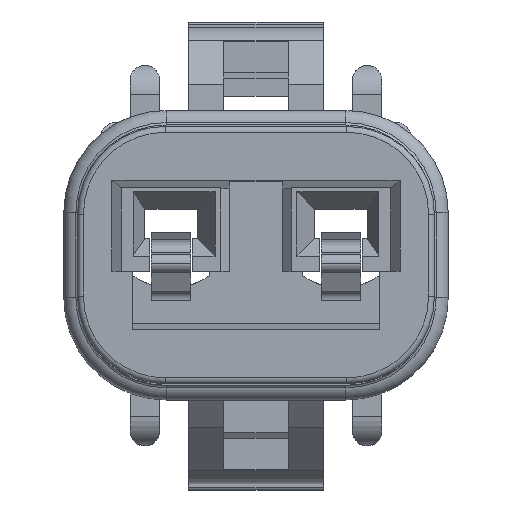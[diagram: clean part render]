
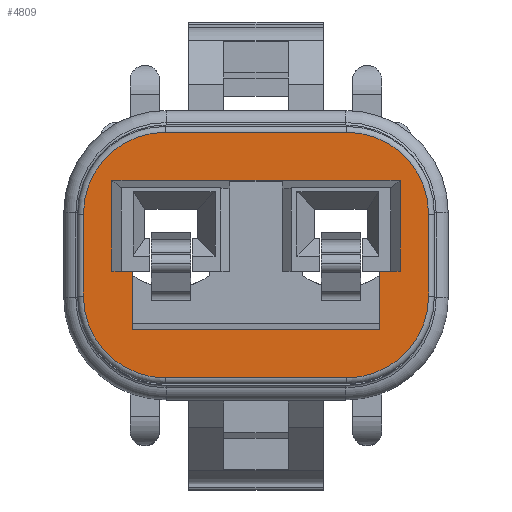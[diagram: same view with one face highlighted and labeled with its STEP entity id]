
A CAD part, top view. The second image highlights one B-rep face of the part: STEP entity #4809.
In plain terms, the highlighted planar face has unit normal (0, 0, 1).
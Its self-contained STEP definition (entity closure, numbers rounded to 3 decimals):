
#49 = ORIENTED_EDGE ( 'NONE', *, *, #10752, .T. ) ;
#76 = ORIENTED_EDGE ( 'NONE', *, *, #14027, .T. ) ;
#453 = CARTESIAN_POINT ( 'NONE',  ( -4.925, 2.55, 1.2 ) ) ;
#725 = DIRECTION ( 'NONE',  ( 0., -1., 0. ) ) ;
#781 = VERTEX_POINT ( 'NONE', #19091 ) ;
#872 = FACE_OUTER_BOUND ( 'NONE', #15510, .T. ) ;
#918 = CIRCLE ( 'NONE', #20754, 2.8 ) ;
#1000 = LINE ( 'NONE', #7420, #5694 ) ;
#1250 = DIRECTION ( 'NONE',  ( 0., 1., 0. ) ) ;
#1324 = VERTEX_POINT ( 'NONE', #19499 ) ;
#1380 = DIRECTION ( 'NONE',  ( -1., 0., 0. ) ) ;
#1539 = DIRECTION ( 'NONE',  ( 0., 1., 0. ) ) ;
#1746 = VERTEX_POINT ( 'NONE', #6311 ) ;
#1815 = VERTEX_POINT ( 'NONE', #8735 ) ;
#2242 = ORIENTED_EDGE ( 'NONE', *, *, #15572, .T. ) ;
#2269 = EDGE_CURVE ( 'NONE', #15715, #1746, #9987, .T. ) ;
#2289 = DIRECTION ( 'NONE',  ( -1., 0., 0. ) ) ;
#2416 = EDGE_CURVE ( 'NONE', #15825, #19016, #18409, .T. ) ;
#2464 = DIRECTION ( 'NONE',  ( 0., -1., 0. ) ) ;
#2472 = DIRECTION ( 'NONE',  ( 0., 0., 1. ) ) ;
#2514 = CARTESIAN_POINT ( 'NONE',  ( -3.1, -1.4, 1.2 ) ) ;
#2639 = CARTESIAN_POINT ( 'NONE',  ( 3.1, 4.2, 1.2 ) ) ;
#2837 = AXIS2_PLACEMENT_3D ( 'NONE', #20809, #11456, #12719 ) ;
#3070 = LINE ( 'NONE', #6118, #18614 ) ;
#3193 = CARTESIAN_POINT ( 'NONE',  ( 3.1, 4.2, 1.2 ) ) ;
#3314 = CARTESIAN_POINT ( 'NONE',  ( 3.1, -4.2, 1.2 ) ) ;
#3358 = CARTESIAN_POINT ( 'NONE',  ( -0.9, 2.55, 1.2 ) ) ;
#3387 = LINE ( 'NONE', #9812, #15746 ) ;
#3481 = EDGE_LOOP ( 'NONE', ( #18229, #16703, #19898, #76, #18916, #15585, #14771, #2242, #17295, #3567 ) ) ;
#3567 = ORIENTED_EDGE ( 'NONE', *, *, #6371, .T. ) ;
#3836 = DIRECTION ( 'NONE',  ( 1., 0., 0. ) ) ;
#4118 = EDGE_CURVE ( 'NONE', #15641, #1815, #9157, .T. ) ;
#4176 = VERTEX_POINT ( 'NONE', #8186 ) ;
#4182 = CARTESIAN_POINT ( 'NONE',  ( -4.225, -0.55, 1.2 ) ) ;
#4259 = AXIS2_PLACEMENT_3D ( 'NONE', #2514, #10612, #16950 ) ;
#4262 = CARTESIAN_POINT ( 'NONE',  ( 0., 0., 1.2 ) ) ;
#4807 = CARTESIAN_POINT ( 'NONE',  ( -4.225, -2.55, 1.2 ) ) ;
#4809 = ADVANCED_FACE ( 'NONE', ( #15211, #872 ), #9203, .T. ) ;
#4913 = VERTEX_POINT ( 'NONE', #3193 ) ;
#5470 = VECTOR ( 'NONE', #20482, 1000. ) ;
#5694 = VECTOR ( 'NONE', #2289, 1000. ) ;
#5737 = EDGE_CURVE ( 'NONE', #781, #15825, #15977, .T. ) ;
#5860 = DIRECTION ( 'NONE',  ( -1., 0., 0. ) ) ;
#5917 = LINE ( 'NONE', #10461, #13371 ) ;
#6086 = CARTESIAN_POINT ( 'NONE',  ( -4.925, -0.55, 1.2 ) ) ;
#6118 = CARTESIAN_POINT ( 'NONE',  ( 4.925, -0.55, 1.2 ) ) ;
#6308 = DIRECTION ( 'NONE',  ( 0., -1., 0. ) ) ;
#6311 = CARTESIAN_POINT ( 'NONE',  ( 0.9, 2.55, 1.2 ) ) ;
#6320 = CARTESIAN_POINT ( 'NONE',  ( -0.9, 2.55, 1.2 ) ) ;
#6371 = EDGE_CURVE ( 'NONE', #17735, #781, #5917, .T. ) ;
#6386 = CARTESIAN_POINT ( 'NONE',  ( -3.1, 4.2, 1.2 ) ) ;
#6433 = EDGE_CURVE ( 'NONE', #1815, #4913, #918, .T. ) ;
#6452 = ORIENTED_EDGE ( 'NONE', *, *, #6433, .T. ) ;
#6667 = EDGE_CURVE ( 'NONE', #1324, #19016, #3387, .T. ) ;
#6841 = ORIENTED_EDGE ( 'NONE', *, *, #9318, .T. ) ;
#7092 = CARTESIAN_POINT ( 'NONE',  ( -3.1, -4.2, 1.2 ) ) ;
#7420 = CARTESIAN_POINT ( 'NONE',  ( 4.925, 2.55, 1.2 ) ) ;
#7669 = EDGE_CURVE ( 'NONE', #9952, #4176, #18721, .T. ) ;
#8186 = CARTESIAN_POINT ( 'NONE',  ( -3.1, -4.2, 1.2 ) ) ;
#8634 = VERTEX_POINT ( 'NONE', #15010 ) ;
#8735 = CARTESIAN_POINT ( 'NONE',  ( 5.9, 1.4, 1.2 ) ) ;
#8788 = CARTESIAN_POINT ( 'NONE',  ( 4.925, 2.55, 1.2 ) ) ;
#8792 = LINE ( 'NONE', #7092, #18320 ) ;
#8938 = CARTESIAN_POINT ( 'NONE',  ( -5.9, -1.4, 1.2 ) ) ;
#9010 = CARTESIAN_POINT ( 'NONE',  ( -5.9, 1.4, 1.2 ) ) ;
#9157 = LINE ( 'NONE', #10839, #15659 ) ;
#9203 = PLANE ( 'NONE',  #9647 ) ;
#9318 = EDGE_CURVE ( 'NONE', #19410, #9952, #17803, .T. ) ;
#9647 = AXIS2_PLACEMENT_3D ( 'NONE', #4262, #2472, #13732 ) ;
#9810 = ORIENTED_EDGE ( 'NONE', *, *, #7669, .T. ) ;
#9812 = CARTESIAN_POINT ( 'NONE',  ( -4.925, 2.55, 1.2 ) ) ;
#9952 = VERTEX_POINT ( 'NONE', #8938 ) ;
#9987 = LINE ( 'NONE', #3358, #11718 ) ;
#10063 = VECTOR ( 'NONE', #1380, 1000. ) ;
#10341 = EDGE_CURVE ( 'NONE', #12966, #1746, #1000, .T. ) ;
#10403 = VECTOR ( 'NONE', #3836, 1000. ) ;
#10461 = CARTESIAN_POINT ( 'NONE',  ( 4.225, -2.55, 1.2 ) ) ;
#10612 = DIRECTION ( 'NONE',  ( 0., 0., 1. ) ) ;
#10713 = VERTEX_POINT ( 'NONE', #3314 ) ;
#10752 = EDGE_CURVE ( 'NONE', #10713, #15641, #11735, .T. ) ;
#10797 = CARTESIAN_POINT ( 'NONE',  ( 4.225, -0.55, 1.2 ) ) ;
#10839 = CARTESIAN_POINT ( 'NONE',  ( 5.9, -1.4, 1.2 ) ) ;
#10959 = LINE ( 'NONE', #2639, #10063 ) ;
#11046 = ORIENTED_EDGE ( 'NONE', *, *, #20813, .T. ) ;
#11456 = DIRECTION ( 'NONE',  ( 0., 0., 1. ) ) ;
#11718 = VECTOR ( 'NONE', #17904, 1000. ) ;
#11735 = CIRCLE ( 'NONE', #14424, 2.8 ) ;
#12140 = DIRECTION ( 'NONE',  ( 0., 0., 1. ) ) ;
#12506 = LINE ( 'NONE', #17343, #5470 ) ;
#12719 = DIRECTION ( 'NONE',  ( 0., 1., 0. ) ) ;
#12966 = VERTEX_POINT ( 'NONE', #8788 ) ;
#13241 = EDGE_CURVE ( 'NONE', #17224, #17735, #15048, .T. ) ;
#13371 = VECTOR ( 'NONE', #18464, 1000. ) ;
#13665 = CARTESIAN_POINT ( 'NONE',  ( -4.225, -0.55, 1.2 ) ) ;
#13732 = DIRECTION ( 'NONE',  ( 1., 0., 0. ) ) ;
#13764 = VECTOR ( 'NONE', #6308, 1000. ) ;
#13976 = ORIENTED_EDGE ( 'NONE', *, *, #20353, .T. ) ;
#14027 = EDGE_CURVE ( 'NONE', #1324, #15715, #18260, .T. ) ;
#14329 = VECTOR ( 'NONE', #1539, 1000. ) ;
#14424 = AXIS2_PLACEMENT_3D ( 'NONE', #15096, #19830, #2464 ) ;
#14771 = ORIENTED_EDGE ( 'NONE', *, *, #14881, .T. ) ;
#14881 = EDGE_CURVE ( 'NONE', #12966, #8634, #12506, .T. ) ;
#15010 = CARTESIAN_POINT ( 'NONE',  ( 4.925, -0.55, 1.2 ) ) ;
#15048 = LINE ( 'NONE', #15162, #17101 ) ;
#15096 = CARTESIAN_POINT ( 'NONE',  ( 3.1, -1.4, 1.2 ) ) ;
#15162 = CARTESIAN_POINT ( 'NONE',  ( 4.225, -0.55, 1.2 ) ) ;
#15189 = ORIENTED_EDGE ( 'NONE', *, *, #19771, .T. ) ;
#15211 = FACE_BOUND ( 'NONE', #3481, .T. ) ;
#15508 = ORIENTED_EDGE ( 'NONE', *, *, #4118, .T. ) ;
#15510 = EDGE_LOOP ( 'NONE', ( #6452, #15189, #13976, #6841, #9810, #11046, #49, #15508 ) ) ;
#15572 = EDGE_CURVE ( 'NONE', #8634, #17224, #3070, .T. ) ;
#15585 = ORIENTED_EDGE ( 'NONE', *, *, #10341, .F. ) ;
#15641 = VERTEX_POINT ( 'NONE', #20537 ) ;
#15659 = VECTOR ( 'NONE', #1250, 1000. ) ;
#15715 = VERTEX_POINT ( 'NONE', #6320 ) ;
#15746 = VECTOR ( 'NONE', #16237, 1000. ) ;
#15825 = VERTEX_POINT ( 'NONE', #4182 ) ;
#15922 = DIRECTION ( 'NONE',  ( -1., 0., 0. ) ) ;
#15977 = LINE ( 'NONE', #4807, #14329 ) ;
#16237 = DIRECTION ( 'NONE',  ( 0., -1., 0. ) ) ;
#16703 = ORIENTED_EDGE ( 'NONE', *, *, #2416, .T. ) ;
#16800 = DIRECTION ( 'NONE',  ( 1., 0., 0. ) ) ;
#16836 = VERTEX_POINT ( 'NONE', #6386 ) ;
#16950 = DIRECTION ( 'NONE',  ( -1., 0., 0. ) ) ;
#17101 = VECTOR ( 'NONE', #725, 1000. ) ;
#17224 = VERTEX_POINT ( 'NONE', #10797 ) ;
#17295 = ORIENTED_EDGE ( 'NONE', *, *, #13241, .T. ) ;
#17343 = CARTESIAN_POINT ( 'NONE',  ( 4.925, 2.55, 1.2 ) ) ;
#17735 = VERTEX_POINT ( 'NONE', #17929 ) ;
#17803 = LINE ( 'NONE', #20726, #13764 ) ;
#17904 = DIRECTION ( 'NONE',  ( 1., 0., 0. ) ) ;
#17929 = CARTESIAN_POINT ( 'NONE',  ( 4.225, -2.55, 1.2 ) ) ;
#18229 = ORIENTED_EDGE ( 'NONE', *, *, #5737, .T. ) ;
#18260 = LINE ( 'NONE', #453, #10403 ) ;
#18320 = VECTOR ( 'NONE', #16800, 1000. ) ;
#18409 = LINE ( 'NONE', #13665, #20776 ) ;
#18464 = DIRECTION ( 'NONE',  ( -1., 0., 0. ) ) ;
#18564 = DIRECTION ( 'NONE',  ( 1., 0., 0. ) ) ;
#18614 = VECTOR ( 'NONE', #15922, 1000. ) ;
#18721 = CIRCLE ( 'NONE', #4259, 2.8 ) ;
#18916 = ORIENTED_EDGE ( 'NONE', *, *, #2269, .T. ) ;
#19016 = VERTEX_POINT ( 'NONE', #6086 ) ;
#19091 = CARTESIAN_POINT ( 'NONE',  ( -4.225, -2.55, 1.2 ) ) ;
#19410 = VERTEX_POINT ( 'NONE', #9010 ) ;
#19499 = CARTESIAN_POINT ( 'NONE',  ( -4.925, 2.55, 1.2 ) ) ;
#19771 = EDGE_CURVE ( 'NONE', #4913, #16836, #10959, .T. ) ;
#19830 = DIRECTION ( 'NONE',  ( 0., 0., 1. ) ) ;
#19898 = ORIENTED_EDGE ( 'NONE', *, *, #6667, .F. ) ;
#20129 = CARTESIAN_POINT ( 'NONE',  ( 3.1, 1.4, 1.2 ) ) ;
#20353 = EDGE_CURVE ( 'NONE', #16836, #19410, #20651, .T. ) ;
#20482 = DIRECTION ( 'NONE',  ( 0., -1., 0. ) ) ;
#20537 = CARTESIAN_POINT ( 'NONE',  ( 5.9, -1.4, 1.2 ) ) ;
#20651 = CIRCLE ( 'NONE', #2837, 2.8 ) ;
#20726 = CARTESIAN_POINT ( 'NONE',  ( -5.9, 1.4, 1.2 ) ) ;
#20754 = AXIS2_PLACEMENT_3D ( 'NONE', #20129, #12140, #18564 ) ;
#20776 = VECTOR ( 'NONE', #5860, 1000. ) ;
#20809 = CARTESIAN_POINT ( 'NONE',  ( -3.1, 1.4, 1.2 ) ) ;
#20813 = EDGE_CURVE ( 'NONE', #4176, #10713, #8792, .T. ) ;
